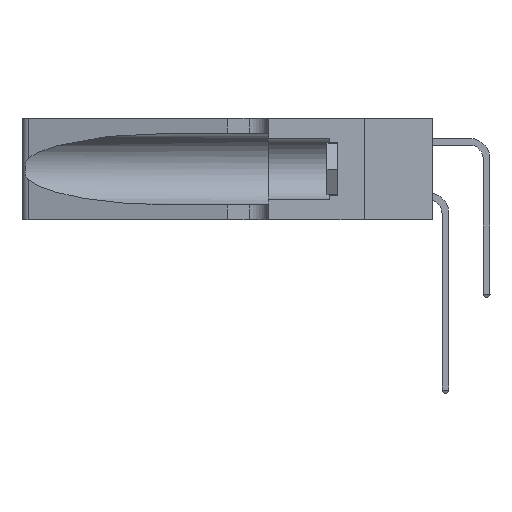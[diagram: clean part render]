
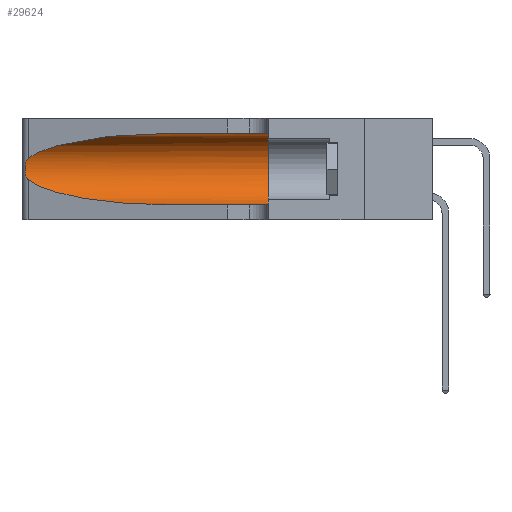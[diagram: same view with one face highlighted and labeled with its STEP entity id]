
A CAD part, left-side view. The second image highlights one B-rep face of the part: STEP entity #29624.
In plain terms, the highlighted cylindrical face has radius 3.308 mm (diameter 6.617 mm), a partial arc.
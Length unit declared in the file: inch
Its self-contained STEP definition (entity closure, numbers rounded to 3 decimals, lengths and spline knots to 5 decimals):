
#383 = CARTESIAN_POINT ( 'NONE',  ( 0.25487, 1.22718, 0.14631 ) ) ;
#1201 = CARTESIAN_POINT ( 'NONE',  ( 0.26075, 1.23896, 0.19203 ) ) ;
#1651 = CARTESIAN_POINT ( 'NONE',  ( 0.1305, 0.72297, 0.05475 ) ) ;
#2931 = CARTESIAN_POINT ( 'NONE',  ( 0.1305, 1.61858, 0.185 ) ) ;
#3271 = CARTESIAN_POINT ( 'NONE',  ( 0.1305, 1.61858, 0.31525 ) ) ;
#4559 = EDGE_CURVE ( 'NONE', #36272, #19774, #37118, .T. ) ;
#4601 = DIRECTION ( 'NONE',  ( 0., -1., 0. ) ) ;
#4795 = CARTESIAN_POINT ( 'NONE',  ( 0.26017, 1.23833, 0.17102 ) ) ;
#5450 = CARTESIAN_POINT ( 'NONE',  ( 0.18966, 0.96281, 0.31525 ) ) ;
#6244 = DIRECTION ( 'NONE',  ( 0., 1., 0. ) ) ;
#8201 = CARTESIAN_POINT ( 'NONE',  ( 0.25555, 1.22994, 0.2215 ) ) ;
#8350 = CARTESIAN_POINT ( 'NONE',  ( 0.25789, 1.23486, 0.15765 ) ) ;
#9160 = CARTESIAN_POINT ( 'NONE',  ( 0.2373, 1.15595, 0.28018 ) ) ;
#10257 = DIRECTION ( 'NONE',  ( 0., 0., -1. ) ) ;
#10788 = VERTEX_POINT ( 'NONE', #45060 ) ;
#11134 = CARTESIAN_POINT ( 'NONE',  ( 0.1305, 0.72297, 0.05475 ) ) ;
#11476 = FACE_OUTER_BOUND ( 'NONE', #16047, .T. ) ;
#11913 = CARTESIAN_POINT ( 'NONE',  ( 0.25555, 1.22993, 0.14849 ) ) ;
#12949 = ORIENTED_EDGE ( 'NONE', *, *, #17394, .T. ) ;
#13918 = EDGE_CURVE ( 'NONE', #16066, #10788, #41068, .T. ) ;
#15012 = EDGE_CURVE ( 'NONE', #32037, #36272, #34869, .T. ) ;
#16047 = EDGE_LOOP ( 'NONE', ( #31984, #35299, #12949, #26063, #19157, #18169 ) ) ;
#16058 = VECTOR ( 'NONE', #4601, 39.37008 ) ;
#16066 = VERTEX_POINT ( 'NONE', #18021 ) ;
#16883 =( BOUNDED_CURVE ( )  B_SPLINE_CURVE ( 3, ( #383, #21555, #32016, #11134 ),
 .UNSPECIFIED., .F., .F. ) 
 B_SPLINE_CURVE_WITH_KNOTS ( ( 4, 4 ),
 ( 3.44316, 4.71239 ),
 .UNSPECIFIED. ) 
 CURVE ( )  GEOMETRIC_REPRESENTATION_ITEM ( )  RATIONAL_B_SPLINE_CURVE ( ( 1., 0.87, 0.87, 1. ) ) 
 REPRESENTATION_ITEM ( '' )  );
#17394 = EDGE_CURVE ( 'NONE', #10788, #34253, #16883, .T. ) ;
#18021 = CARTESIAN_POINT ( 'NONE',  ( 0.25487, 1.22718, 0.22369 ) ) ;
#18169 = ORIENTED_EDGE ( 'NONE', *, *, #15012, .F. ) ;
#18859 = CARTESIAN_POINT ( 'NONE',  ( 0.25787, 1.23484, 0.2124 ) ) ;
#19157 = ORIENTED_EDGE ( 'NONE', *, *, #4559, .F. ) ;
#19774 = VERTEX_POINT ( 'NONE', #22172 ) ;
#21555 = CARTESIAN_POINT ( 'NONE',  ( 0.2373, 1.15595, 0.08982 ) ) ;
#22172 = CARTESIAN_POINT ( 'NONE',  ( 0.1305, 0.35, 0.05475 ) ) ;
#22351 = CARTESIAN_POINT ( 'NONE',  ( 0.26018, 1.23835, 0.19895 ) ) ;
#23132 = CARTESIAN_POINT ( 'NONE',  ( 0.1305, 0.72297, 0.31525 ) ) ;
#23978 = EDGE_CURVE ( 'NONE', #34253, #19774, #44772, .T. ) ;
#25833 = CARTESIAN_POINT ( 'NONE',  ( 0.26075, 1.23896, 0.178 ) ) ;
#26063 = ORIENTED_EDGE ( 'NONE', *, *, #23978, .T. ) ;
#27296 = CARTESIAN_POINT ( 'NONE',  ( 0.1305, 0.35, 0.185 ) ) ;
#29330 = CARTESIAN_POINT ( 'NONE',  ( 0.25856, 1.23593, 0.16098 ) ) ;
#29485 = AXIS2_PLACEMENT_3D ( 'NONE', #27296, #6244, #30746 ) ;
#29624 = ADVANCED_FACE ( 'NONE', ( #11476 ), #37104, .F. ) ;
#30746 = DIRECTION ( 'NONE',  ( 0., 0., 1. ) ) ;
#31131 = DIRECTION ( 'NONE',  ( 0., -1., 0. ) ) ;
#31984 = ORIENTED_EDGE ( 'NONE', *, *, #35313, .T. ) ;
#32016 = CARTESIAN_POINT ( 'NONE',  ( 0.18966, 0.96281, 0.05475 ) ) ;
#32037 = VERTEX_POINT ( 'NONE', #41849 ) ;
#32640 = CARTESIAN_POINT ( 'NONE',  ( 0.25487, 1.22718, 0.22369 ) ) ;
#32793 = CARTESIAN_POINT ( 'NONE',  ( 0.25639, 1.23186, 0.15144 ) ) ;
#33564 = CARTESIAN_POINT ( 'NONE',  ( 0.25487, 1.22718, 0.22369 ) ) ;
#33782 = VECTOR ( 'NONE', #45027, 39.37008 ) ;
#33990 = AXIS2_PLACEMENT_3D ( 'NONE', #2931, #31131, #10257 ) ;
#34253 = VERTEX_POINT ( 'NONE', #1651 ) ;
#34869 = LINE ( 'NONE', #3271, #33782 ) ;
#35299 = ORIENTED_EDGE ( 'NONE', *, *, #13918, .T. ) ;
#35313 = EDGE_CURVE ( 'NONE', #32037, #16066, #42440, .T. ) ;
#36272 = VERTEX_POINT ( 'NONE', #41941 ) ;
#36308 = CARTESIAN_POINT ( 'NONE',  ( 0.25487, 1.22718, 0.14631 ) ) ;
#37104 = CYLINDRICAL_SURFACE ( 'NONE', #33990, 0.13025 ) ;
#37118 = CIRCLE ( 'NONE', #29485, 0.13025 ) ;
#39427 = CARTESIAN_POINT ( 'NONE',  ( 0.1305, 1.61858, 0.05475 ) ) ;
#39610 = CARTESIAN_POINT ( 'NONE',  ( 0.25639, 1.23184, 0.21858 ) ) ;
#41068 = B_SPLINE_CURVE_WITH_KNOTS ( 'NONE', 3,
 ( #32640, #8201, #39610, #18859, #43043, #22351, #1201, #25833, #4795, #29330, #8350, #32793, #11913, #36308 ),
 .UNSPECIFIED., .F., .F.,
 ( 4, 2, 2, 2, 2, 2, 4 ),
 ( 0., 0.00027, 0.00053, 0.00107, 0.0016, 0.00187, 0.00214 ),
 .UNSPECIFIED. ) ;
#41849 = CARTESIAN_POINT ( 'NONE',  ( 0.1305, 0.72297, 0.31525 ) ) ;
#41941 = CARTESIAN_POINT ( 'NONE',  ( 0.1305, 0.35, 0.31525 ) ) ;
#42440 =( BOUNDED_CURVE ( )  B_SPLINE_CURVE ( 3, ( #23132, #5450, #9160, #33564 ),
 .UNSPECIFIED., .F., .F. ) 
 B_SPLINE_CURVE_WITH_KNOTS ( ( 4, 4 ),
 ( 1.5708, 2.84003 ),
 .UNSPECIFIED. ) 
 CURVE ( )  GEOMETRIC_REPRESENTATION_ITEM ( )  RATIONAL_B_SPLINE_CURVE ( ( 1., 0.87, 0.87, 1. ) ) 
 REPRESENTATION_ITEM ( '' )  );
#43043 = CARTESIAN_POINT ( 'NONE',  ( 0.25854, 1.2359, 0.20912 ) ) ;
#44772 = LINE ( 'NONE', #39427, #16058 ) ;
#45027 = DIRECTION ( 'NONE',  ( 0., -1., 0. ) ) ;
#45060 = CARTESIAN_POINT ( 'NONE',  ( 0.25487, 1.22718, 0.14631 ) ) ;
